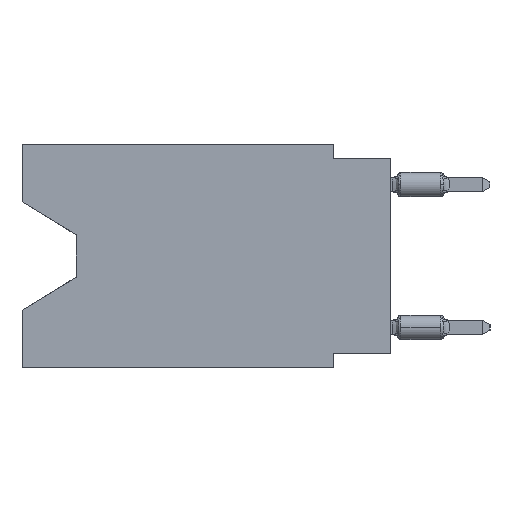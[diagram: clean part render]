
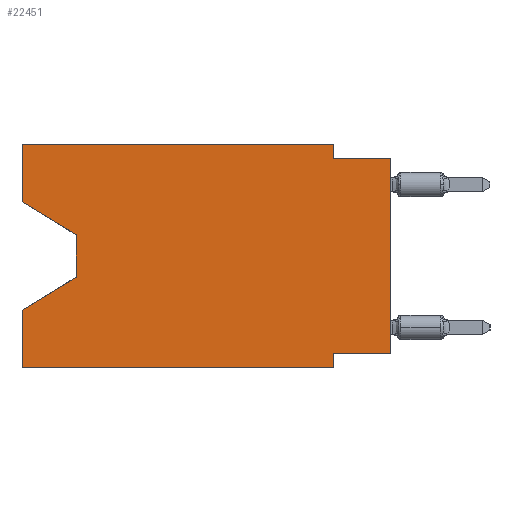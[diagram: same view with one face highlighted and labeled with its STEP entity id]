
A CAD part, left-side view. The second image highlights one B-rep face of the part: STEP entity #22451.
In plain terms, the highlighted planar face has unit normal (-1, 0, 0).
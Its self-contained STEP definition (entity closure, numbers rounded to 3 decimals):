
#918 = DIRECTION ( 'NONE',  ( 0., -0.855, -0.519 ) ) ;
#1089 = CARTESIAN_POINT ( 'NONE',  ( 0., 16.383, -9.906 ) ) ;
#2053 = EDGE_CURVE ( 'NONE', #39360, #4717, #8267, .T. ) ;
#2125 = EDGE_CURVE ( 'NONE', #58885, #22138, #41483, .T. ) ;
#3793 = CARTESIAN_POINT ( 'NONE',  ( 0., 0., -0.635 ) ) ;
#3962 = EDGE_CURVE ( 'NONE', #31016, #4717, #37069, .T. ) ;
#3963 = ORIENTED_EDGE ( 'NONE', *, *, #49747, .F. ) ;
#4547 = ORIENTED_EDGE ( 'NONE', *, *, #16673, .F. ) ;
#4552 = LINE ( 'NONE', #17176, #14371 ) ;
#4717 = VERTEX_POINT ( 'NONE', #55182 ) ;
#5008 = DIRECTION ( 'NONE',  ( 0., 0., 1. ) ) ;
#5687 = CARTESIAN_POINT ( 'NONE',  ( 0., 0., 0. ) ) ;
#5882 = FACE_OUTER_BOUND ( 'NONE', #42285, .T. ) ;
#6443 = CARTESIAN_POINT ( 'NONE',  ( 0., 16.383, -9.906 ) ) ;
#6585 = AXIS2_PLACEMENT_3D ( 'NONE', #29857, #46907, #23876 ) ;
#7212 = VECTOR ( 'NONE', #7409, 1000. ) ;
#7409 = DIRECTION ( 'NONE',  ( 0., -1., 0. ) ) ;
#7702 = CARTESIAN_POINT ( 'NONE',  ( 0., 16.383, 0. ) ) ;
#8266 = EDGE_CURVE ( 'NONE', #11632, #58885, #32096, .T. ) ;
#8267 = LINE ( 'NONE', #26536, #18697 ) ;
#8885 = CARTESIAN_POINT ( 'NONE',  ( 0., 13.97, -4.013 ) ) ;
#10109 = DIRECTION ( 'NONE',  ( 0., -1., 0. ) ) ;
#10311 = CARTESIAN_POINT ( 'NONE',  ( 0., 2.54, 0. ) ) ;
#11318 = LINE ( 'NONE', #7702, #56301 ) ;
#11632 = VERTEX_POINT ( 'NONE', #57214 ) ;
#14127 = VECTOR ( 'NONE', #24034, 1000. ) ;
#14239 = DIRECTION ( 'NONE',  ( 0., 0., -1. ) ) ;
#14371 = VECTOR ( 'NONE', #35718, 1000. ) ;
#15791 = VERTEX_POINT ( 'NONE', #32686 ) ;
#16673 = EDGE_CURVE ( 'NONE', #31016, #28032, #27774, .T. ) ;
#17009 = LINE ( 'NONE', #3793, #7212 ) ;
#17176 = CARTESIAN_POINT ( 'NONE',  ( 0., 0., -9.271 ) ) ;
#17552 = VECTOR ( 'NONE', #42003, 1000. ) ;
#17915 = ORIENTED_EDGE ( 'NONE', *, *, #55418, .T. ) ;
#18350 = CARTESIAN_POINT ( 'NONE',  ( 0., 16.383, -2.546 ) ) ;
#18697 = VECTOR ( 'NONE', #45376, 1000. ) ;
#19263 = CARTESIAN_POINT ( 'NONE',  ( 0., 13.97, -5.893 ) ) ;
#21512 = ORIENTED_EDGE ( 'NONE', *, *, #35822, .F. ) ;
#22138 = VERTEX_POINT ( 'NONE', #33513 ) ;
#22451 = ADVANCED_FACE ( 'NONE', ( #5882 ), #33448, .F. ) ;
#23876 = DIRECTION ( 'NONE',  ( 0., 0., -1. ) ) ;
#24034 = DIRECTION ( 'NONE',  ( 0., 0., -1. ) ) ;
#24400 = CARTESIAN_POINT ( 'NONE',  ( 0., 13.97, -4.013 ) ) ;
#24546 = VERTEX_POINT ( 'NONE', #34534 ) ;
#25019 = CARTESIAN_POINT ( 'NONE',  ( 0., 2.54, -9.271 ) ) ;
#25193 = ORIENTED_EDGE ( 'NONE', *, *, #8266, .T. ) ;
#26536 = CARTESIAN_POINT ( 'NONE',  ( 0., 2.54, -9.906 ) ) ;
#27774 = LINE ( 'NONE', #46036, #53143 ) ;
#28032 = VERTEX_POINT ( 'NONE', #37465 ) ;
#28061 = ORIENTED_EDGE ( 'NONE', *, *, #29066, .F. ) ;
#28379 = CARTESIAN_POINT ( 'NONE',  ( 0., 16.383, 0. ) ) ;
#28518 = CARTESIAN_POINT ( 'NONE',  ( 0., 2.54, 0. ) ) ;
#29066 = EDGE_CURVE ( 'NONE', #45146, #39360, #4552, .T. ) ;
#29857 = CARTESIAN_POINT ( 'NONE',  ( 0., 16.383, 0. ) ) ;
#31016 = VERTEX_POINT ( 'NONE', #6443 ) ;
#32096 = LINE ( 'NONE', #18350, #57481 ) ;
#32686 = CARTESIAN_POINT ( 'NONE',  ( 0., 0., -0.635 ) ) ;
#32897 = ORIENTED_EDGE ( 'NONE', *, *, #54999, .T. ) ;
#33240 = DIRECTION ( 'NONE',  ( 0., 0., 1. ) ) ;
#33448 = PLANE ( 'NONE',  #6585 ) ;
#33513 = CARTESIAN_POINT ( 'NONE',  ( 0., 13.97, -5.893 ) ) ;
#34534 = CARTESIAN_POINT ( 'NONE',  ( 0., 2.54, -0.635 ) ) ;
#35718 = DIRECTION ( 'NONE',  ( 0., 1., 0. ) ) ;
#35822 = EDGE_CURVE ( 'NONE', #43126, #48090, #56823, .T. ) ;
#37041 = EDGE_CURVE ( 'NONE', #24546, #15791, #17009, .T. ) ;
#37069 = LINE ( 'NONE', #1089, #48639 ) ;
#37465 = CARTESIAN_POINT ( 'NONE',  ( 0., 16.383, -7.36 ) ) ;
#38704 = VECTOR ( 'NONE', #10109, 1000. ) ;
#38839 = ORIENTED_EDGE ( 'NONE', *, *, #2053, .F. ) ;
#38949 = EDGE_CURVE ( 'NONE', #11632, #43126, #11318, .T. ) ;
#39001 = ORIENTED_EDGE ( 'NONE', *, *, #3962, .T. ) ;
#39360 = VERTEX_POINT ( 'NONE', #25019 ) ;
#39462 = DIRECTION ( 'NONE',  ( 0., 0., 1. ) ) ;
#39862 = ORIENTED_EDGE ( 'NONE', *, *, #37041, .F. ) ;
#41483 = LINE ( 'NONE', #24400, #56942 ) ;
#41971 = ORIENTED_EDGE ( 'NONE', *, *, #38949, .F. ) ;
#42003 = DIRECTION ( 'NONE',  ( 0., 0.855, -0.519 ) ) ;
#42285 = EDGE_LOOP ( 'NONE', ( #25193, #48563, #32897, #4547, #39001, #38839, #28061, #17915, #39862, #3963, #21512, #41971 ) ) ;
#42441 = VECTOR ( 'NONE', #33240, 1000. ) ;
#43126 = VERTEX_POINT ( 'NONE', #51692 ) ;
#45146 = VERTEX_POINT ( 'NONE', #54885 ) ;
#45376 = DIRECTION ( 'NONE',  ( 0., 0., -1. ) ) ;
#46036 = CARTESIAN_POINT ( 'NONE',  ( 0., 16.383, 0. ) ) ;
#46782 = LINE ( 'NONE', #19263, #17552 ) ;
#46907 = DIRECTION ( 'NONE',  ( 1., 0., 0. ) ) ;
#48090 = VERTEX_POINT ( 'NONE', #10311 ) ;
#48563 = ORIENTED_EDGE ( 'NONE', *, *, #2125, .T. ) ;
#48639 = VECTOR ( 'NONE', #51116, 1000. ) ;
#49747 = EDGE_CURVE ( 'NONE', #48090, #24546, #50388, .T. ) ;
#50388 = LINE ( 'NONE', #28518, #14127 ) ;
#51116 = DIRECTION ( 'NONE',  ( 0., -1., 0. ) ) ;
#51193 = LINE ( 'NONE', #5687, #42441 ) ;
#51692 = CARTESIAN_POINT ( 'NONE',  ( 0., 16.383, 0. ) ) ;
#53143 = VECTOR ( 'NONE', #5008, 1000. ) ;
#54885 = CARTESIAN_POINT ( 'NONE',  ( 0., 0., -9.271 ) ) ;
#54999 = EDGE_CURVE ( 'NONE', #22138, #28032, #46782, .T. ) ;
#55182 = CARTESIAN_POINT ( 'NONE',  ( 0., 2.54, -9.906 ) ) ;
#55418 = EDGE_CURVE ( 'NONE', #45146, #15791, #51193, .T. ) ;
#56301 = VECTOR ( 'NONE', #39462, 1000. ) ;
#56823 = LINE ( 'NONE', #28379, #38704 ) ;
#56942 = VECTOR ( 'NONE', #14239, 1000. ) ;
#57214 = CARTESIAN_POINT ( 'NONE',  ( 0., 16.383, -2.546 ) ) ;
#57481 = VECTOR ( 'NONE', #918, 1000. ) ;
#58885 = VERTEX_POINT ( 'NONE', #8885 ) ;
